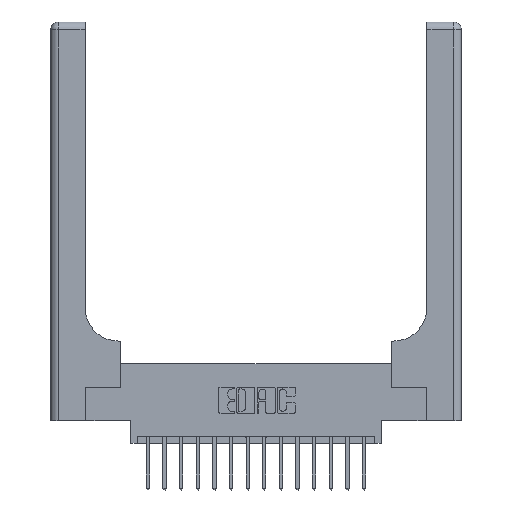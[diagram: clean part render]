
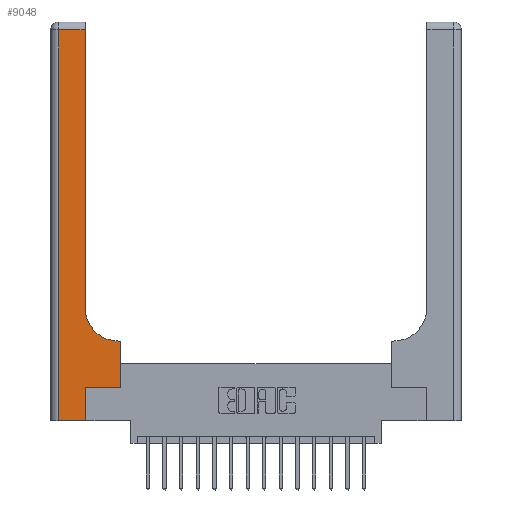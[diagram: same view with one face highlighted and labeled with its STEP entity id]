
A CAD part, top view. The second image highlights one B-rep face of the part: STEP entity #9048.
In plain terms, the highlighted planar face has unit normal (0, 0, 1).
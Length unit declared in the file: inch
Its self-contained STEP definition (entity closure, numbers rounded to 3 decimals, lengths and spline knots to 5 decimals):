
#46 = CARTESIAN_POINT ( 'NONE',  ( 0., 0., 0.37 ) ) ;
#394 = LINE ( 'NONE', #14827, #3680 ) ;
#573 = CIRCLE ( 'NONE', #4348, 0.25 ) ;
#702 = DIRECTION ( 'NONE',  ( -1., 0., 0. ) ) ;
#854 = DIRECTION ( 'NONE',  ( 0., 0., -1. ) ) ;
#1173 = CARTESIAN_POINT ( 'NONE',  ( 0., 2.94, 0.37 ) ) ;
#1660 = CARTESIAN_POINT ( 'NONE',  ( 0.06, 2.94, 0.37 ) ) ;
#1665 = ORIENTED_EDGE ( 'NONE', *, *, #17778, .T. ) ;
#1800 = CARTESIAN_POINT ( 'NONE',  ( 0.265, 0., 0.37 ) ) ;
#1855 = CARTESIAN_POINT ( 'NONE',  ( 0.06, 3., 0.37 ) ) ;
#1866 = LINE ( 'NONE', #1800, #5171 ) ;
#2788 = CARTESIAN_POINT ( 'NONE',  ( 0.26, 0.85, 0.37 ) ) ;
#2998 = EDGE_CURVE ( 'NONE', #5899, #10539, #1866, .T. ) ;
#3247 = DIRECTION ( 'NONE',  ( 0., -1., 0. ) ) ;
#3292 = CARTESIAN_POINT ( 'NONE',  ( 0.528, 0.25, 0.37 ) ) ;
#3533 = VERTEX_POINT ( 'NONE', #14474 ) ;
#3680 = VECTOR ( 'NONE', #702, 39.37008 ) ;
#4085 = DIRECTION ( 'NONE',  ( 1., 0., 0. ) ) ;
#4226 = ORIENTED_EDGE ( 'NONE', *, *, #9777, .T. ) ;
#4348 = AXIS2_PLACEMENT_3D ( 'NONE', #9311, #854, #10733 ) ;
#4807 = ORIENTED_EDGE ( 'NONE', *, *, #2998, .T. ) ;
#4995 = VECTOR ( 'NONE', #11278, 39.37008 ) ;
#5018 = VERTEX_POINT ( 'NONE', #12023 ) ;
#5171 = VECTOR ( 'NONE', #15941, 39.37008 ) ;
#5235 = VECTOR ( 'NONE', #15079, 39.37008 ) ;
#5425 = ORIENTED_EDGE ( 'NONE', *, *, #8585, .T. ) ;
#5684 = LINE ( 'NONE', #13633, #5235 ) ;
#5887 = DIRECTION ( 'NONE',  ( -1., 0., 0. ) ) ;
#5899 = VERTEX_POINT ( 'NONE', #6875 ) ;
#6158 = CARTESIAN_POINT ( 'NONE',  ( 0.51, 0.6, 0.37 ) ) ;
#6871 = VECTOR ( 'NONE', #4085, 39.37008 ) ;
#6875 = CARTESIAN_POINT ( 'NONE',  ( 0.265, 0., 0.37 ) ) ;
#7707 = CARTESIAN_POINT ( 'NONE',  ( 0.265, 0.25, 0.37 ) ) ;
#8073 = CARTESIAN_POINT ( 'NONE',  ( 0.528, 0.6, 0.37 ) ) ;
#8585 = EDGE_CURVE ( 'NONE', #3533, #9386, #13746, .T. ) ;
#8768 = ORIENTED_EDGE ( 'NONE', *, *, #15199, .T. ) ;
#9048 = ADVANCED_FACE ( 'NONE', ( #10883 ), #11496, .F. ) ;
#9311 = CARTESIAN_POINT ( 'NONE',  ( 0.51, 0.85, 0.37 ) ) ;
#9386 = VERTEX_POINT ( 'NONE', #8073 ) ;
#9723 = CARTESIAN_POINT ( 'NONE',  ( 0.06, 0., 0.37 ) ) ;
#9777 = EDGE_CURVE ( 'NONE', #14163, #15191, #11073, .T. ) ;
#10453 = VECTOR ( 'NONE', #17450, 39.37008 ) ;
#10539 = VERTEX_POINT ( 'NONE', #7707 ) ;
#10630 = LINE ( 'NONE', #13899, #6871 ) ;
#10733 = DIRECTION ( 'NONE',  ( 1., 0., 0. ) ) ;
#10883 = FACE_OUTER_BOUND ( 'NONE', #16417, .T. ) ;
#10903 = EDGE_CURVE ( 'NONE', #15191, #5899, #16771, .T. ) ;
#11073 = LINE ( 'NONE', #1855, #18122 ) ;
#11278 = DIRECTION ( 'NONE',  ( -1., 0., 0. ) ) ;
#11496 = PLANE ( 'NONE',  #12113 ) ;
#12023 = CARTESIAN_POINT ( 'NONE',  ( 0.26, 2.94, 0.37 ) ) ;
#12113 = AXIS2_PLACEMENT_3D ( 'NONE', #12915, #14335, #5887 ) ;
#12327 = ORIENTED_EDGE ( 'NONE', *, *, #18161, .T. ) ;
#12724 = DIRECTION ( 'NONE',  ( 1., 0., 0. ) ) ;
#12833 = ORIENTED_EDGE ( 'NONE', *, *, #17046, .T. ) ;
#12915 = CARTESIAN_POINT ( 'NONE',  ( 0., 3., 0.37 ) ) ;
#12973 = VERTEX_POINT ( 'NONE', #2788 ) ;
#12999 = VECTOR ( 'NONE', #12724, 39.37008 ) ;
#13633 = CARTESIAN_POINT ( 'NONE',  ( 0.26, 3., 0.37 ) ) ;
#13746 = LINE ( 'NONE', #3292, #10453 ) ;
#13899 = CARTESIAN_POINT ( 'NONE',  ( 0.265, 0.25, 0.37 ) ) ;
#14163 = VERTEX_POINT ( 'NONE', #1660 ) ;
#14335 = DIRECTION ( 'NONE',  ( 0., 0., -1. ) ) ;
#14474 = CARTESIAN_POINT ( 'NONE',  ( 0.528, 0.25, 0.37 ) ) ;
#14827 = CARTESIAN_POINT ( 'NONE',  ( 0.26, 0.6, 0.37 ) ) ;
#14859 = ORIENTED_EDGE ( 'NONE', *, *, #10903, .T. ) ;
#14935 = ORIENTED_EDGE ( 'NONE', *, *, #16938, .T. ) ;
#15079 = DIRECTION ( 'NONE',  ( 0., 1., 0. ) ) ;
#15191 = VERTEX_POINT ( 'NONE', #9723 ) ;
#15199 = EDGE_CURVE ( 'NONE', #10539, #3533, #10630, .T. ) ;
#15819 = LINE ( 'NONE', #1173, #4995 ) ;
#15941 = DIRECTION ( 'NONE',  ( 0., 1., 0. ) ) ;
#16417 = EDGE_LOOP ( 'NONE', ( #12833, #1665, #4226, #14859, #4807, #8768, #5425, #14935, #12327 ) ) ;
#16771 = LINE ( 'NONE', #46, #12999 ) ;
#16938 = EDGE_CURVE ( 'NONE', #9386, #18006, #394, .T. ) ;
#17046 = EDGE_CURVE ( 'NONE', #12973, #5018, #5684, .T. ) ;
#17450 = DIRECTION ( 'NONE',  ( 0., 1., 0. ) ) ;
#17778 = EDGE_CURVE ( 'NONE', #5018, #14163, #15819, .T. ) ;
#18006 = VERTEX_POINT ( 'NONE', #6158 ) ;
#18122 = VECTOR ( 'NONE', #3247, 39.37008 ) ;
#18161 = EDGE_CURVE ( 'NONE', #18006, #12973, #573, .T. ) ;
